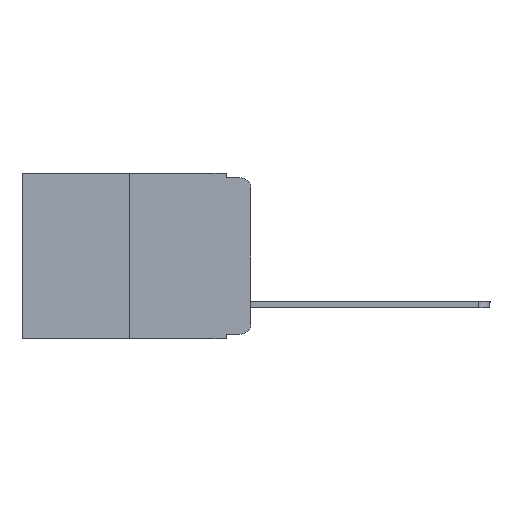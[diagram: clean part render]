
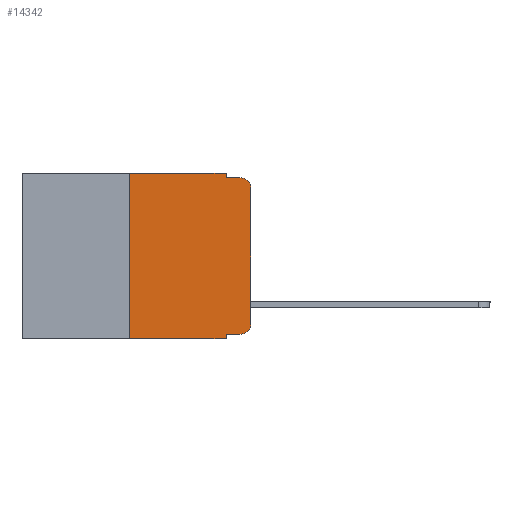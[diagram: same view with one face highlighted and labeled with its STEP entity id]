
A CAD part, left-side view. The second image highlights one B-rep face of the part: STEP entity #14342.
In plain terms, the highlighted planar face has unit normal (-1, 0, 0).
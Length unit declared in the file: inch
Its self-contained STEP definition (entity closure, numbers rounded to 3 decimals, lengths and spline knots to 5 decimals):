
#190 = DIRECTION ( 'NONE',  ( 0., 0., -1. ) ) ;
#238 = CARTESIAN_POINT ( 'NONE',  ( 0., 0.051, 0. ) ) ;
#380 = VERTEX_POINT ( 'NONE', #6272 ) ;
#538 = CARTESIAN_POINT ( 'NONE',  ( 0., 0.051, 0. ) ) ;
#836 = VECTOR ( 'NONE', #10013, 39.37008 ) ;
#1005 = EDGE_CURVE ( 'NONE', #9285, #14613, #8184, .T. ) ;
#1344 = EDGE_CURVE ( 'NONE', #12119, #16946, #20927, .T. ) ;
#1908 = EDGE_CURVE ( 'NONE', #14236, #14770, #11745, .T. ) ;
#2605 = VECTOR ( 'NONE', #15241, 39.37008 ) ;
#3375 = VERTEX_POINT ( 'NONE', #16516 ) ;
#3560 = CARTESIAN_POINT ( 'NONE',  ( 0., 0.25, 0. ) ) ;
#3661 = AXIS2_PLACEMENT_3D ( 'NONE', #14019, #9037, #20422 ) ;
#4050 = EDGE_CURVE ( 'NONE', #380, #3375, #17009, .T. ) ;
#4447 = EDGE_CURVE ( 'NONE', #16090, #12119, #14680, .T. ) ;
#4466 = CARTESIAN_POINT ( 'NONE',  ( 0., 0.051, -0.333 ) ) ;
#4625 = ORIENTED_EDGE ( 'NONE', *, *, #4447, .F. ) ;
#4667 = CARTESIAN_POINT ( 'NONE',  ( 0., 0.25, -0.343 ) ) ;
#5114 = CARTESIAN_POINT ( 'NONE',  ( 0., 0.051, -0.343 ) ) ;
#5260 = ORIENTED_EDGE ( 'NONE', *, *, #17155, .T. ) ;
#5440 = DIRECTION ( 'NONE',  ( 0., 0., -1. ) ) ;
#5542 = FACE_OUTER_BOUND ( 'NONE', #14688, .T. ) ;
#5764 = ORIENTED_EDGE ( 'NONE', *, *, #6328, .T. ) ;
#6066 = ORIENTED_EDGE ( 'NONE', *, *, #8353, .F. ) ;
#6272 = CARTESIAN_POINT ( 'NONE',  ( 0., 0.051, -0.01 ) ) ;
#6328 = EDGE_CURVE ( 'NONE', #14770, #3375, #14211, .T. ) ;
#6350 = CARTESIAN_POINT ( 'NONE',  ( 0., 0.02, -0.333 ) ) ;
#6704 = DIRECTION ( 'NONE',  ( 0., 0., -1. ) ) ;
#7025 = ORIENTED_EDGE ( 'NONE', *, *, #1005, .F. ) ;
#7327 = CARTESIAN_POINT ( 'NONE',  ( 0., 0., -0.03 ) ) ;
#7926 = CARTESIAN_POINT ( 'NONE',  ( 0., 0.051, -0.01 ) ) ;
#8128 = ORIENTED_EDGE ( 'NONE', *, *, #4050, .F. ) ;
#8184 = LINE ( 'NONE', #238, #18576 ) ;
#8333 = AXIS2_PLACEMENT_3D ( 'NONE', #11809, #20198, #5440 ) ;
#8353 = EDGE_CURVE ( 'NONE', #16946, #380, #8491, .T. ) ;
#8491 = LINE ( 'NONE', #538, #12291 ) ;
#9037 = DIRECTION ( 'NONE',  ( 1., 0., 0. ) ) ;
#9285 = VERTEX_POINT ( 'NONE', #10688 ) ;
#9549 = DIRECTION ( 'NONE',  ( 0., -1., 0. ) ) ;
#9908 = CARTESIAN_POINT ( 'NONE',  ( 0., 0., -0.313 ) ) ;
#10013 = DIRECTION ( 'NONE',  ( 0., 0., 1. ) ) ;
#10095 = CARTESIAN_POINT ( 'NONE',  ( 0., 0.051, 0. ) ) ;
#10688 = CARTESIAN_POINT ( 'NONE',  ( 0., 0.051, -0.333 ) ) ;
#10855 = DIRECTION ( 'NONE',  ( 0., -1., 0. ) ) ;
#11426 = ORIENTED_EDGE ( 'NONE', *, *, #1344, .F. ) ;
#11745 = LINE ( 'NONE', #11853, #2605 ) ;
#11809 = CARTESIAN_POINT ( 'NONE',  ( 0., 0.02, -0.313 ) ) ;
#11844 = AXIS2_PLACEMENT_3D ( 'NONE', #16726, #14714, #190 ) ;
#11853 = CARTESIAN_POINT ( 'NONE',  ( 0., 0., 0. ) ) ;
#12119 = VERTEX_POINT ( 'NONE', #17353 ) ;
#12291 = VECTOR ( 'NONE', #16362, 39.37008 ) ;
#13166 = ORIENTED_EDGE ( 'NONE', *, *, #18279, .T. ) ;
#13233 = VECTOR ( 'NONE', #17409, 39.37008 ) ;
#13823 = PLANE ( 'NONE',  #3661 ) ;
#14019 = CARTESIAN_POINT ( 'NONE',  ( 0., 0.473, 0. ) ) ;
#14211 = CIRCLE ( 'NONE', #11844, 0.02 ) ;
#14236 = VERTEX_POINT ( 'NONE', #9908 ) ;
#14342 = ADVANCED_FACE ( 'NONE', ( #5542 ), #13823, .F. ) ;
#14613 = VERTEX_POINT ( 'NONE', #5114 ) ;
#14680 = LINE ( 'NONE', #3560, #836 ) ;
#14688 = EDGE_LOOP ( 'NONE', ( #17904, #5764, #8128, #6066, #11426, #4625, #15049, #7025, #5260, #13166 ) ) ;
#14714 = DIRECTION ( 'NONE',  ( -1., 0., 0. ) ) ;
#14770 = VERTEX_POINT ( 'NONE', #7327 ) ;
#14773 = VECTOR ( 'NONE', #17492, 39.37008 ) ;
#15049 = ORIENTED_EDGE ( 'NONE', *, *, #20964, .T. ) ;
#15241 = DIRECTION ( 'NONE',  ( 0., 0., 1. ) ) ;
#16090 = VERTEX_POINT ( 'NONE', #4667 ) ;
#16242 = CARTESIAN_POINT ( 'NONE',  ( 0., 0.473, 0. ) ) ;
#16362 = DIRECTION ( 'NONE',  ( 0., 0., -1. ) ) ;
#16516 = CARTESIAN_POINT ( 'NONE',  ( 0., 0.02, -0.01 ) ) ;
#16726 = CARTESIAN_POINT ( 'NONE',  ( 0., 0.02, -0.03 ) ) ;
#16946 = VERTEX_POINT ( 'NONE', #10095 ) ;
#17009 = LINE ( 'NONE', #7926, #14773 ) ;
#17155 = EDGE_CURVE ( 'NONE', #9285, #20370, #19031, .T. ) ;
#17353 = CARTESIAN_POINT ( 'NONE',  ( 0., 0.25, 0. ) ) ;
#17409 = DIRECTION ( 'NONE',  ( 0., -1., 0. ) ) ;
#17492 = DIRECTION ( 'NONE',  ( 0., -1., 0. ) ) ;
#17904 = ORIENTED_EDGE ( 'NONE', *, *, #1908, .T. ) ;
#18279 = EDGE_CURVE ( 'NONE', #20370, #14236, #19540, .T. ) ;
#18576 = VECTOR ( 'NONE', #6704, 39.37008 ) ;
#18945 = CARTESIAN_POINT ( 'NONE',  ( 0., 0.473, -0.343 ) ) ;
#19031 = LINE ( 'NONE', #4466, #13233 ) ;
#19278 = VECTOR ( 'NONE', #10855, 39.37008 ) ;
#19540 = CIRCLE ( 'NONE', #8333, 0.02 ) ;
#20198 = DIRECTION ( 'NONE',  ( -1., 0., 0. ) ) ;
#20370 = VERTEX_POINT ( 'NONE', #6350 ) ;
#20422 = DIRECTION ( 'NONE',  ( 0., 0., -1. ) ) ;
#20436 = VECTOR ( 'NONE', #9549, 39.37008 ) ;
#20531 = LINE ( 'NONE', #18945, #19278 ) ;
#20927 = LINE ( 'NONE', #16242, #20436 ) ;
#20964 = EDGE_CURVE ( 'NONE', #16090, #14613, #20531, .T. ) ;
